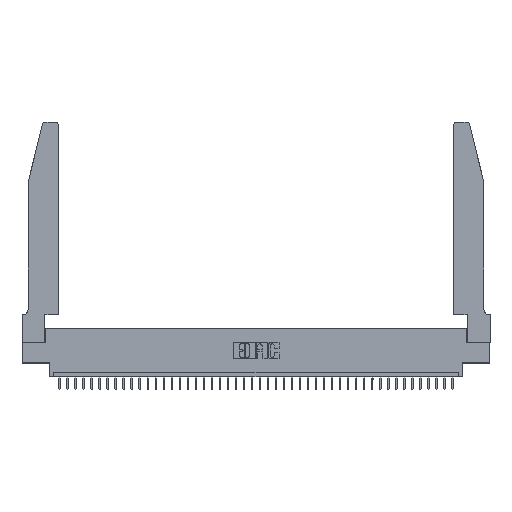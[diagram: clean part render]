
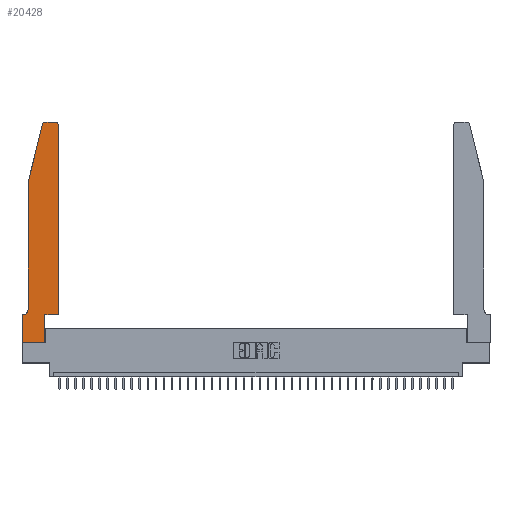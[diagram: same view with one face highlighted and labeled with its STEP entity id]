
A CAD part, top view. The second image highlights one B-rep face of the part: STEP entity #20428.
In plain terms, the highlighted planar face has unit normal (0, 0, 1).
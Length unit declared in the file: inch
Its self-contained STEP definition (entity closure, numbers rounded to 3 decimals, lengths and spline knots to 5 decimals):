
#380 = CARTESIAN_POINT ( 'NONE',  ( 0.0755, 0.35, 0.37 ) ) ;
#626 = VERTEX_POINT ( 'NONE', #41153 ) ;
#1579 = DIRECTION ( 'NONE',  ( 1., 0., 0. ) ) ;
#2702 = ORIENTED_EDGE ( 'NONE', *, *, #22729, .T. ) ;
#2801 = DIRECTION ( 'NONE',  ( 0., -1., 0. ) ) ;
#3055 = EDGE_CURVE ( 'NONE', #626, #11441, #6573, .T. ) ;
#3286 = EDGE_CURVE ( 'NONE', #31193, #626, #10531, .T. ) ;
#3871 = EDGE_CURVE ( 'NONE', #37793, #32590, #22382, .T. ) ;
#3872 = EDGE_CURVE ( 'NONE', #16094, #37793, #39966, .T. ) ;
#3942 = DIRECTION ( 'NONE',  ( -1., 0., 0. ) ) ;
#4197 = CARTESIAN_POINT ( 'NONE',  ( 0.2865, 0.35, 0.37 ) ) ;
#4894 = AXIS2_PLACEMENT_3D ( 'NONE', #40468, #36471, #7902 ) ;
#5000 = ORIENTED_EDGE ( 'NONE', *, *, #16395, .T. ) ;
#5408 = LINE ( 'NONE', #380, #33880 ) ;
#6131 = VECTOR ( 'NONE', #2801, 39.37008 ) ;
#6573 = LINE ( 'NONE', #28075, #6131 ) ;
#6955 = CIRCLE ( 'NONE', #27975, 0.07 ) ;
#7292 = VERTEX_POINT ( 'NONE', #8030 ) ;
#7758 = VERTEX_POINT ( 'NONE', #9960 ) ;
#7902 = DIRECTION ( 'NONE',  ( 1., 0., 0. ) ) ;
#8030 = CARTESIAN_POINT ( 'NONE',  ( 0.0055, 0.35, 0.37 ) ) ;
#8108 = VECTOR ( 'NONE', #12044, 39.37008 ) ;
#8348 = ORIENTED_EDGE ( 'NONE', *, *, #13949, .T. ) ;
#9035 = CARTESIAN_POINT ( 'NONE',  ( 0., 0., 0.37 ) ) ;
#9398 = CIRCLE ( 'NONE', #14189, 0.03 ) ;
#9477 = VECTOR ( 'NONE', #15274, 39.37008 ) ;
#9766 = ORIENTED_EDGE ( 'NONE', *, *, #3286, .T. ) ;
#9960 = CARTESIAN_POINT ( 'NONE',  ( 0.4205, 2.75, 0.37 ) ) ;
#10321 = EDGE_CURVE ( 'NONE', #7758, #17385, #22930, .T. ) ;
#10531 = LINE ( 'NONE', #37336, #36520 ) ;
#10850 = CARTESIAN_POINT ( 'NONE',  ( 0.2865, 0.35, 0.37 ) ) ;
#11288 = CARTESIAN_POINT ( 'NONE',  ( 0., 0.35, 0.37 ) ) ;
#11441 = VERTEX_POINT ( 'NONE', #16825 ) ;
#11646 = AXIS2_PLACEMENT_3D ( 'NONE', #33445, #33152, #33596 ) ;
#11747 = CARTESIAN_POINT ( 'NONE',  ( 0.2605, 2.75, 0.37 ) ) ;
#12044 = DIRECTION ( 'NONE',  ( -1., 0., 0. ) ) ;
#12400 = ORIENTED_EDGE ( 'NONE', *, *, #3871, .T. ) ;
#12883 = CARTESIAN_POINT ( 'NONE',  ( 0.4505, 0.35, 0.37 ) ) ;
#13210 = ORIENTED_EDGE ( 'NONE', *, *, #10321, .T. ) ;
#13949 = EDGE_CURVE ( 'NONE', #19140, #27993, #39768, .T. ) ;
#14189 = AXIS2_PLACEMENT_3D ( 'NONE', #17359, #14762, #37120 ) ;
#14286 = EDGE_CURVE ( 'NONE', #27993, #16094, #33722, .T. ) ;
#14762 = DIRECTION ( 'NONE',  ( 0., 0., 1. ) ) ;
#14861 = CARTESIAN_POINT ( 'NONE',  ( 0.4505, 2.72, 0.37 ) ) ;
#15274 = DIRECTION ( 'NONE',  ( 0., -1., 0. ) ) ;
#16094 = VERTEX_POINT ( 'NONE', #4197 ) ;
#16395 = EDGE_CURVE ( 'NONE', #32590, #7758, #9398, .T. ) ;
#16825 = CARTESIAN_POINT ( 'NONE',  ( 0.0755, 0.42, 0.37 ) ) ;
#17359 = CARTESIAN_POINT ( 'NONE',  ( 0.4205, 2.72, 0.37 ) ) ;
#17369 = CARTESIAN_POINT ( 'NONE',  ( 0., 0., 0.37 ) ) ;
#17385 = VERTEX_POINT ( 'NONE', #38940 ) ;
#17846 = LINE ( 'NONE', #9035, #9477 ) ;
#18588 = DIRECTION ( 'NONE',  ( -1., 0., 0. ) ) ;
#19140 = VERTEX_POINT ( 'NONE', #17369 ) ;
#19387 = VECTOR ( 'NONE', #35298, 39.37008 ) ;
#19510 = EDGE_CURVE ( 'NONE', #17385, #31193, #31974, .T. ) ;
#20428 = ADVANCED_FACE ( 'NONE', ( #31453 ), #22102, .T. ) ;
#21327 = DIRECTION ( 'NONE',  ( -0.239, -0.971, 0. ) ) ;
#21760 = CARTESIAN_POINT ( 'NONE',  ( 0.0055, 0.42, 0.37 ) ) ;
#21894 = DIRECTION ( 'NONE',  ( 0., 0., -1. ) ) ;
#22102 = PLANE ( 'NONE',  #4894 ) ;
#22382 = LINE ( 'NONE', #31445, #36440 ) ;
#22729 = EDGE_CURVE ( 'NONE', #11441, #7292, #6955, .T. ) ;
#22780 = CARTESIAN_POINT ( 'NONE',  ( 0., 0., 0.37 ) ) ;
#22930 = LINE ( 'NONE', #11747, #8108 ) ;
#23580 = CARTESIAN_POINT ( 'NONE',  ( 0.4505, 0.35, 0.37 ) ) ;
#26627 = ORIENTED_EDGE ( 'NONE', *, *, #14286, .T. ) ;
#27975 = AXIS2_PLACEMENT_3D ( 'NONE', #21760, #21894, #18588 ) ;
#27993 = VERTEX_POINT ( 'NONE', #35370 ) ;
#28075 = CARTESIAN_POINT ( 'NONE',  ( 0.0755, 2., 0.37 ) ) ;
#28235 = ORIENTED_EDGE ( 'NONE', *, *, #3055, .T. ) ;
#30005 = CARTESIAN_POINT ( 'NONE',  ( 0.25487, 2.72718, 0.37 ) ) ;
#31193 = VERTEX_POINT ( 'NONE', #30005 ) ;
#31445 = CARTESIAN_POINT ( 'NONE',  ( 0.4505, 0.35, 0.37 ) ) ;
#31453 = FACE_OUTER_BOUND ( 'NONE', #38112, .T. ) ;
#31974 = CIRCLE ( 'NONE', #11646, 0.03 ) ;
#32590 = VERTEX_POINT ( 'NONE', #14861 ) ;
#32702 = VECTOR ( 'NONE', #1579, 39.37008 ) ;
#33152 = DIRECTION ( 'NONE',  ( 0., 0., 1. ) ) ;
#33298 = DIRECTION ( 'NONE',  ( 0., 1., 0. ) ) ;
#33445 = CARTESIAN_POINT ( 'NONE',  ( 0.284, 2.72, 0.37 ) ) ;
#33596 = DIRECTION ( 'NONE',  ( 1., 0., 0. ) ) ;
#33722 = LINE ( 'NONE', #10850, #40798 ) ;
#33880 = VECTOR ( 'NONE', #3942, 39.37008 ) ;
#35298 = DIRECTION ( 'NONE',  ( 1., 0., 0. ) ) ;
#35370 = CARTESIAN_POINT ( 'NONE',  ( 0.2865, 0., 0.37 ) ) ;
#35900 = ORIENTED_EDGE ( 'NONE', *, *, #37619, .T. ) ;
#36144 = ORIENTED_EDGE ( 'NONE', *, *, #36788, .T. ) ;
#36440 = VECTOR ( 'NONE', #38041, 39.37008 ) ;
#36471 = DIRECTION ( 'NONE',  ( 0., 0., 1. ) ) ;
#36520 = VECTOR ( 'NONE', #21327, 39.37008 ) ;
#36657 = ORIENTED_EDGE ( 'NONE', *, *, #3872, .T. ) ;
#36788 = EDGE_CURVE ( 'NONE', #41205, #19140, #17846, .T. ) ;
#37032 = ORIENTED_EDGE ( 'NONE', *, *, #19510, .T. ) ;
#37120 = DIRECTION ( 'NONE',  ( 1., 0., 0. ) ) ;
#37336 = CARTESIAN_POINT ( 'NONE',  ( 0.0755, 2., 0.37 ) ) ;
#37619 = EDGE_CURVE ( 'NONE', #7292, #41205, #5408, .T. ) ;
#37793 = VERTEX_POINT ( 'NONE', #23580 ) ;
#38041 = DIRECTION ( 'NONE',  ( 0., 1., 0. ) ) ;
#38112 = EDGE_LOOP ( 'NONE', ( #13210, #37032, #9766, #28235, #2702, #35900, #36144, #8348, #26627, #36657, #12400, #5000 ) ) ;
#38940 = CARTESIAN_POINT ( 'NONE',  ( 0.284, 2.75, 0.37 ) ) ;
#39768 = LINE ( 'NONE', #22780, #32702 ) ;
#39966 = LINE ( 'NONE', #12883, #19387 ) ;
#40468 = CARTESIAN_POINT ( 'NONE',  ( 0., 0.35, 0.37 ) ) ;
#40798 = VECTOR ( 'NONE', #33298, 39.37008 ) ;
#41153 = CARTESIAN_POINT ( 'NONE',  ( 0.0755, 2., 0.37 ) ) ;
#41205 = VERTEX_POINT ( 'NONE', #11288 ) ;
